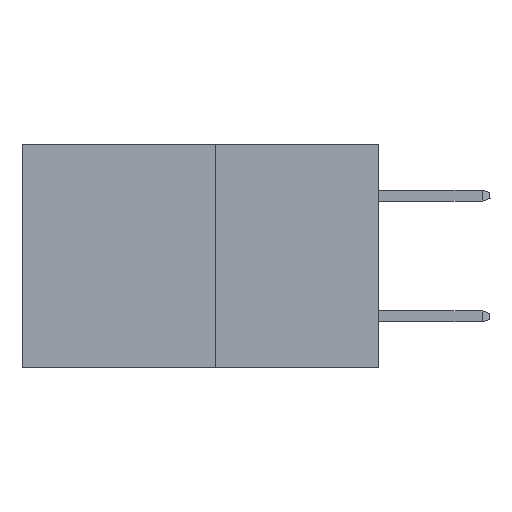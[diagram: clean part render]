
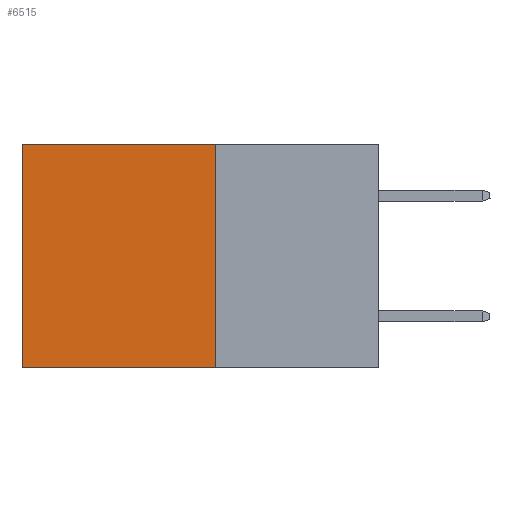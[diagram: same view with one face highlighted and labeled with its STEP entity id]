
A CAD part, left-side view. The second image highlights one B-rep face of the part: STEP entity #6515.
In plain terms, the highlighted planar face has unit normal (-1, 0, 0).
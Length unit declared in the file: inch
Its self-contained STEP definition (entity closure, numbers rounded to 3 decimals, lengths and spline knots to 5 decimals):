
#676 = VERTEX_POINT ( 'NONE', #680 ) ;
#680 = CARTESIAN_POINT ( 'NONE',  ( 0.277, 0.59, -0.37 ) ) ;
#801 = VECTOR ( 'NONE', #28107, 39.37008 ) ;
#1586 = VERTEX_POINT ( 'NONE', #26455 ) ;
#1667 = CARTESIAN_POINT ( 'NONE',  ( 0.277, 0.59, 0. ) ) ;
#1705 = CARTESIAN_POINT ( 'NONE',  ( 0.277, 0.27, -0.37 ) ) ;
#1797 = ORIENTED_EDGE ( 'NONE', *, *, #22519, .F. ) ;
#3425 = DIRECTION ( 'NONE',  ( 0., 0., -1. ) ) ;
#5639 = ORIENTED_EDGE ( 'NONE', *, *, #22226, .F. ) ;
#6001 = VECTOR ( 'NONE', #26554, 39.37008 ) ;
#6477 = VERTEX_POINT ( 'NONE', #1667 ) ;
#6515 = ADVANCED_FACE ( 'NONE', ( #20418 ), #33881, .F. ) ;
#7957 = AXIS2_PLACEMENT_3D ( 'NONE', #34785, #33649, #33619 ) ;
#9036 = LINE ( 'NONE', #27997, #801 ) ;
#9614 = ORIENTED_EDGE ( 'NONE', *, *, #33269, .T. ) ;
#12408 = LINE ( 'NONE', #23843, #6001 ) ;
#14221 = LINE ( 'NONE', #34913, #23252 ) ;
#18703 = DIRECTION ( 'NONE',  ( 0., 1., 0. ) ) ;
#19895 = CARTESIAN_POINT ( 'NONE',  ( 0.277, 0.59, -0.37 ) ) ;
#20418 = FACE_OUTER_BOUND ( 'NONE', #20867, .T. ) ;
#20787 = EDGE_CURVE ( 'NONE', #6477, #676, #32129, .T. ) ;
#20867 = EDGE_LOOP ( 'NONE', ( #34809, #5639, #1797, #9614 ) ) ;
#21025 = VERTEX_POINT ( 'NONE', #1705 ) ;
#22226 = EDGE_CURVE ( 'NONE', #21025, #676, #9036, .T. ) ;
#22519 = EDGE_CURVE ( 'NONE', #1586, #21025, #12408, .T. ) ;
#23252 = VECTOR ( 'NONE', #18703, 39.37008 ) ;
#23843 = CARTESIAN_POINT ( 'NONE',  ( 0.277, 0.27, -0.37 ) ) ;
#24939 = VECTOR ( 'NONE', #3425, 39.37008 ) ;
#26455 = CARTESIAN_POINT ( 'NONE',  ( 0.277, 0.27, 0. ) ) ;
#26554 = DIRECTION ( 'NONE',  ( 0., 0., -1. ) ) ;
#27997 = CARTESIAN_POINT ( 'NONE',  ( 0.277, 0.27, -0.37 ) ) ;
#28107 = DIRECTION ( 'NONE',  ( 0., 1., 0. ) ) ;
#32129 = LINE ( 'NONE', #19895, #24939 ) ;
#33269 = EDGE_CURVE ( 'NONE', #1586, #6477, #14221, .T. ) ;
#33619 = DIRECTION ( 'NONE',  ( 0., 0., -1. ) ) ;
#33649 = DIRECTION ( 'NONE',  ( 1., 0., 0. ) ) ;
#33881 = PLANE ( 'NONE',  #7957 ) ;
#34785 = CARTESIAN_POINT ( 'NONE',  ( 0.277, 0.27, -0.37 ) ) ;
#34809 = ORIENTED_EDGE ( 'NONE', *, *, #20787, .T. ) ;
#34913 = CARTESIAN_POINT ( 'NONE',  ( 0.277, 0.27, 0. ) ) ;
